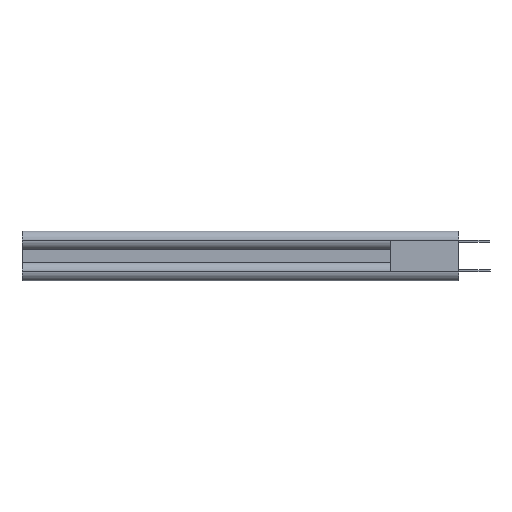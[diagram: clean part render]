
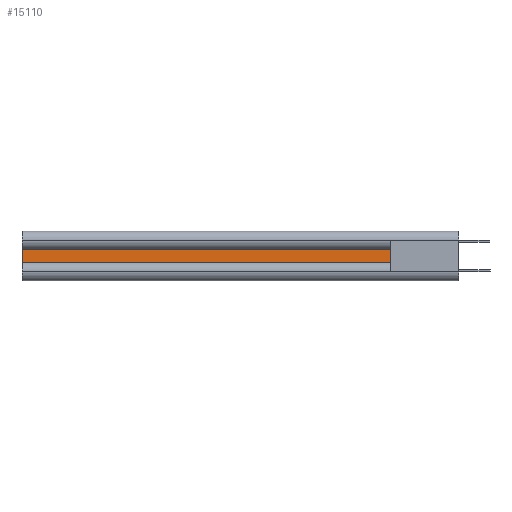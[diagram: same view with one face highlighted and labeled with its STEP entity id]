
A CAD part, left-side view. The second image highlights one B-rep face of the part: STEP entity #15110.
In plain terms, the highlighted planar face has unit normal (-1, 0, 0).
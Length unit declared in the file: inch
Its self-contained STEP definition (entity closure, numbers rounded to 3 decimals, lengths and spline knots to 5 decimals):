
#12 = CARTESIAN_POINT ( 'NONE',  ( 0.044, 0.473, -0.0465 ) ) ;
#266 = EDGE_CURVE ( 'NONE', #14626, #4686, #7024, .T. ) ;
#516 = DIRECTION ( 'NONE',  ( 0., 1., 0. ) ) ;
#668 = VECTOR ( 'NONE', #4472, 39.37008 ) ;
#1151 = VECTOR ( 'NONE', #12158, 39.37008 ) ;
#2595 = DIRECTION ( 'NONE',  ( 0., 0., -1. ) ) ;
#2808 = EDGE_LOOP ( 'NONE', ( #21521, #19917, #3330, #10855 ) ) ;
#3096 = CARTESIAN_POINT ( 'NONE',  ( 0.044, 3., -0.0465 ) ) ;
#3330 = ORIENTED_EDGE ( 'NONE', *, *, #16226, .F. ) ;
#4472 = DIRECTION ( 'NONE',  ( 0., 0., -1. ) ) ;
#4686 = VERTEX_POINT ( 'NONE', #14522 ) ;
#4705 = DIRECTION ( 'NONE',  ( 0., 0., -1. ) ) ;
#5287 = CARTESIAN_POINT ( 'NONE',  ( 0.044, 0.37012, 0.0465 ) ) ;
#5838 = LINE ( 'NONE', #5287, #1151 ) ;
#6298 = EDGE_CURVE ( 'NONE', #14626, #6899, #5838, .T. ) ;
#6483 = VECTOR ( 'NONE', #2595, 39.37008 ) ;
#6899 = VERTEX_POINT ( 'NONE', #10488 ) ;
#7024 = LINE ( 'NONE', #12, #6483 ) ;
#8130 = DIRECTION ( 'NONE',  ( 1., 0., 0. ) ) ;
#9480 = LINE ( 'NONE', #9730, #668 ) ;
#9730 = CARTESIAN_POINT ( 'NONE',  ( 0.044, 3., -0.0465 ) ) ;
#10488 = CARTESIAN_POINT ( 'NONE',  ( 0.044, 3., 0.0465 ) ) ;
#10855 = ORIENTED_EDGE ( 'NONE', *, *, #266, .F. ) ;
#12158 = DIRECTION ( 'NONE',  ( 0., 1., 0. ) ) ;
#13064 = EDGE_CURVE ( 'NONE', #6899, #20378, #9480, .T. ) ;
#13319 = CARTESIAN_POINT ( 'NONE',  ( 0.044, 0.37012, -0.0465 ) ) ;
#14522 = CARTESIAN_POINT ( 'NONE',  ( 0.044, 0.473, -0.0465 ) ) ;
#14626 = VERTEX_POINT ( 'NONE', #17654 ) ;
#15025 = PLANE ( 'NONE',  #20998 ) ;
#15110 = ADVANCED_FACE ( 'NONE', ( #16569 ), #15025, .F. ) ;
#15331 = VECTOR ( 'NONE', #516, 39.37008 ) ;
#15845 = LINE ( 'NONE', #16051, #15331 ) ;
#16051 = CARTESIAN_POINT ( 'NONE',  ( 0.044, 0.37012, -0.0465 ) ) ;
#16226 = EDGE_CURVE ( 'NONE', #4686, #20378, #15845, .T. ) ;
#16569 = FACE_OUTER_BOUND ( 'NONE', #2808, .T. ) ;
#17654 = CARTESIAN_POINT ( 'NONE',  ( 0.044, 0.473, 0.0465 ) ) ;
#19917 = ORIENTED_EDGE ( 'NONE', *, *, #13064, .T. ) ;
#20378 = VERTEX_POINT ( 'NONE', #3096 ) ;
#20998 = AXIS2_PLACEMENT_3D ( 'NONE', #13319, #8130, #4705 ) ;
#21521 = ORIENTED_EDGE ( 'NONE', *, *, #6298, .T. ) ;
